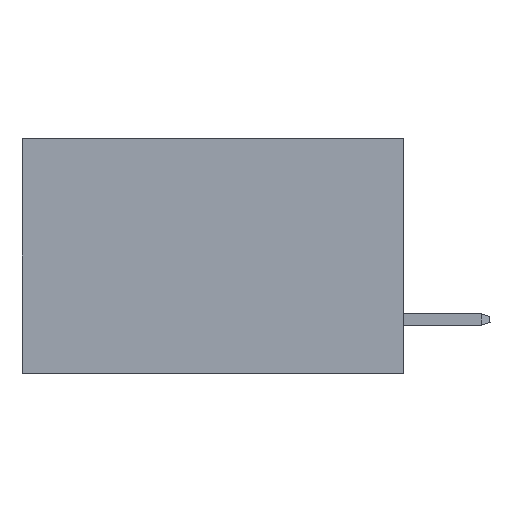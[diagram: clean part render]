
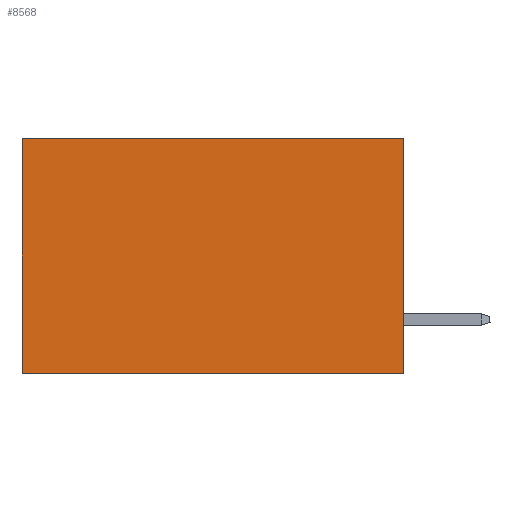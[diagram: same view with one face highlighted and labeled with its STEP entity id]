
A CAD part, left-side view. The second image highlights one B-rep face of the part: STEP entity #8568.
In plain terms, the highlighted planar face has unit normal (-1, 0, 0).
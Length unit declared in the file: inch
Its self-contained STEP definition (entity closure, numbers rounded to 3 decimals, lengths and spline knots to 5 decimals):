
#1587 = ORIENTED_EDGE ( 'NONE', *, *, #6517, .T. ) ;
#2148 = CARTESIAN_POINT ( 'NONE',  ( 0.2875, 0.6, 0. ) ) ;
#2161 = VERTEX_POINT ( 'NONE', #29632 ) ;
#2211 = PLANE ( 'NONE',  #34270 ) ;
#3129 = EDGE_CURVE ( 'NONE', #18042, #20437, #22368, .T. ) ;
#3835 = FACE_OUTER_BOUND ( 'NONE', #15198, .T. ) ;
#6141 = LINE ( 'NONE', #2148, #30887 ) ;
#6517 = EDGE_CURVE ( 'NONE', #12673, #20437, #6141, .T. ) ;
#6739 = LINE ( 'NONE', #18526, #17607 ) ;
#8568 = ADVANCED_FACE ( 'NONE', ( #3835 ), #2211, .F. ) ;
#8593 = EDGE_CURVE ( 'NONE', #2161, #18042, #6739, .T. ) ;
#12673 = VERTEX_POINT ( 'NONE', #33002 ) ;
#12907 = DIRECTION ( 'NONE',  ( 0., 1., 0. ) ) ;
#13051 = VECTOR ( 'NONE', #36367, 39.37008 ) ;
#15198 = EDGE_LOOP ( 'NONE', ( #1587, #16112, #36911, #25593 ) ) ;
#15638 = DIRECTION ( 'NONE',  ( 0., 0., -1. ) ) ;
#15681 = CARTESIAN_POINT ( 'NONE',  ( 0.2875, 0., 0. ) ) ;
#16112 = ORIENTED_EDGE ( 'NONE', *, *, #3129, .F. ) ;
#16728 = CARTESIAN_POINT ( 'NONE',  ( 0.2875, 0., 0. ) ) ;
#17607 = VECTOR ( 'NONE', #15638, 39.37008 ) ;
#18042 = VERTEX_POINT ( 'NONE', #28971 ) ;
#18526 = CARTESIAN_POINT ( 'NONE',  ( 0.2875, 0., 0. ) ) ;
#20437 = VERTEX_POINT ( 'NONE', #34231 ) ;
#21799 = CARTESIAN_POINT ( 'NONE',  ( 0.2875, 0., -0.37 ) ) ;
#22368 = LINE ( 'NONE', #21799, #26035 ) ;
#25593 = ORIENTED_EDGE ( 'NONE', *, *, #31208, .T. ) ;
#26035 = VECTOR ( 'NONE', #12907, 39.37008 ) ;
#28501 = DIRECTION ( 'NONE',  ( 1., 0., 0. ) ) ;
#28971 = CARTESIAN_POINT ( 'NONE',  ( 0.2875, 0., -0.37 ) ) ;
#29005 = DIRECTION ( 'NONE',  ( 0., 0., -1. ) ) ;
#29632 = CARTESIAN_POINT ( 'NONE',  ( 0.2875, 0., 0. ) ) ;
#30887 = VECTOR ( 'NONE', #29005, 39.37008 ) ;
#31208 = EDGE_CURVE ( 'NONE', #2161, #12673, #33825, .T. ) ;
#31396 = DIRECTION ( 'NONE',  ( 0., 0., -1. ) ) ;
#33002 = CARTESIAN_POINT ( 'NONE',  ( 0.2875, 0.6, 0. ) ) ;
#33825 = LINE ( 'NONE', #15681, #13051 ) ;
#34231 = CARTESIAN_POINT ( 'NONE',  ( 0.2875, 0.6, -0.37 ) ) ;
#34270 = AXIS2_PLACEMENT_3D ( 'NONE', #16728, #28501, #31396 ) ;
#36367 = DIRECTION ( 'NONE',  ( 0., 1., 0. ) ) ;
#36911 = ORIENTED_EDGE ( 'NONE', *, *, #8593, .F. ) ;
